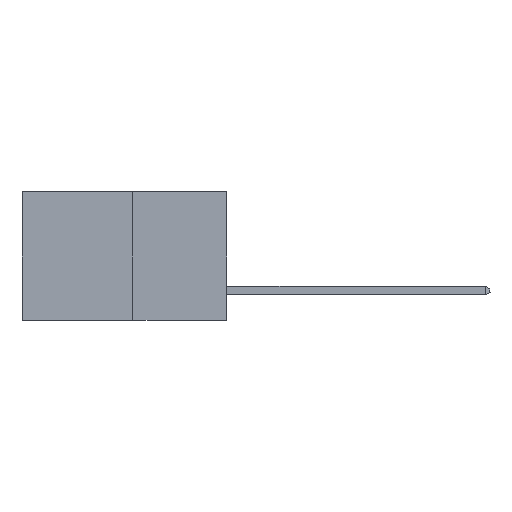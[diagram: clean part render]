
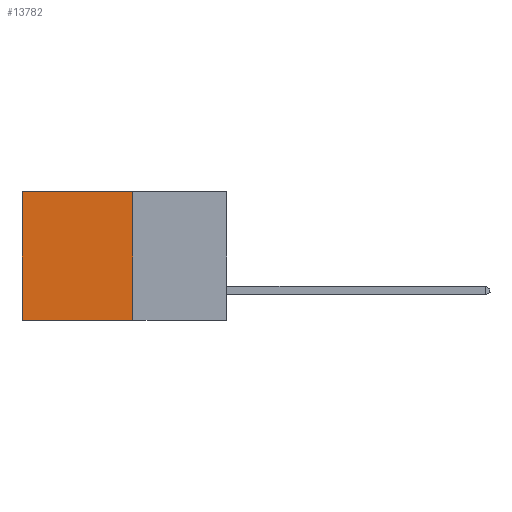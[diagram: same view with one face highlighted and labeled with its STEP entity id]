
A CAD part, left-side view. The second image highlights one B-rep face of the part: STEP entity #13782.
In plain terms, the highlighted planar face has unit normal (-1, 0, 0).
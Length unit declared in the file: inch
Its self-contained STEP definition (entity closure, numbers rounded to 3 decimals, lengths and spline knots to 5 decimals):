
#35 = ORIENTED_EDGE ( 'NONE', *, *, #2698, .T. ) ;
#722 = PLANE ( 'NONE',  #11155 ) ;
#1050 = VECTOR ( 'NONE', #5845, 39.37008 ) ;
#1111 = EDGE_CURVE ( 'NONE', #4639, #12197, #11150, .T. ) ;
#1154 = DIRECTION ( 'NONE',  ( 0., 1., 0. ) ) ;
#2219 = DIRECTION ( 'NONE',  ( 0., 0., -1. ) ) ;
#2323 = EDGE_CURVE ( 'NONE', #4639, #8681, #3618, .T. ) ;
#2425 = VECTOR ( 'NONE', #1154, 39.37008 ) ;
#2698 = EDGE_CURVE ( 'NONE', #12197, #4993, #9924, .T. ) ;
#2766 = LINE ( 'NONE', #5511, #2425 ) ;
#3267 = ORIENTED_EDGE ( 'NONE', *, *, #4151, .F. ) ;
#3601 = CARTESIAN_POINT ( 'NONE',  ( 0.277, 0.27, -0.37 ) ) ;
#3618 = LINE ( 'NONE', #3601, #1050 ) ;
#3825 = EDGE_LOOP ( 'NONE', ( #35, #3267, #11433, #8923 ) ) ;
#4013 = DIRECTION ( 'NONE',  ( 1., 0., 0. ) ) ;
#4151 = EDGE_CURVE ( 'NONE', #8681, #4993, #2766, .T. ) ;
#4639 = VERTEX_POINT ( 'NONE', #10889 ) ;
#4993 = VERTEX_POINT ( 'NONE', #9796 ) ;
#5511 = CARTESIAN_POINT ( 'NONE',  ( 0.277, 0.27, -0.37 ) ) ;
#5845 = DIRECTION ( 'NONE',  ( 0., 0., -1. ) ) ;
#7082 = CARTESIAN_POINT ( 'NONE',  ( 0.277, 0.27, -0.37 ) ) ;
#7783 = VECTOR ( 'NONE', #2219, 39.37008 ) ;
#8336 = VECTOR ( 'NONE', #10923, 39.37008 ) ;
#8487 = CARTESIAN_POINT ( 'NONE',  ( 0.277, 0.59, -0.37 ) ) ;
#8681 = VERTEX_POINT ( 'NONE', #7082 ) ;
#8923 = ORIENTED_EDGE ( 'NONE', *, *, #1111, .T. ) ;
#9796 = CARTESIAN_POINT ( 'NONE',  ( 0.277, 0.59, -0.37 ) ) ;
#9876 = CARTESIAN_POINT ( 'NONE',  ( 0.277, 0.59, 0. ) ) ;
#9924 = LINE ( 'NONE', #8487, #7783 ) ;
#10383 = CARTESIAN_POINT ( 'NONE',  ( 0.277, 0.27, -0.37 ) ) ;
#10703 = CARTESIAN_POINT ( 'NONE',  ( 0.277, 0.27, 0. ) ) ;
#10889 = CARTESIAN_POINT ( 'NONE',  ( 0.277, 0.27, 0. ) ) ;
#10923 = DIRECTION ( 'NONE',  ( 0., 1., 0. ) ) ;
#11150 = LINE ( 'NONE', #10703, #8336 ) ;
#11155 = AXIS2_PLACEMENT_3D ( 'NONE', #10383, #4013, #11481 ) ;
#11433 = ORIENTED_EDGE ( 'NONE', *, *, #2323, .F. ) ;
#11481 = DIRECTION ( 'NONE',  ( 0., 0., -1. ) ) ;
#11884 = FACE_OUTER_BOUND ( 'NONE', #3825, .T. ) ;
#12197 = VERTEX_POINT ( 'NONE', #9876 ) ;
#13782 = ADVANCED_FACE ( 'NONE', ( #11884 ), #722, .F. ) ;
